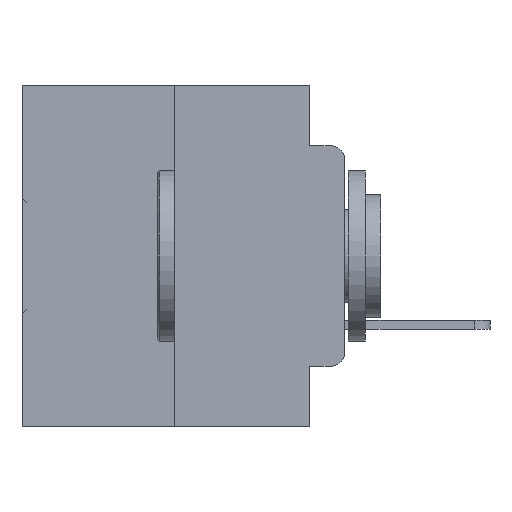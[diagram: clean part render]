
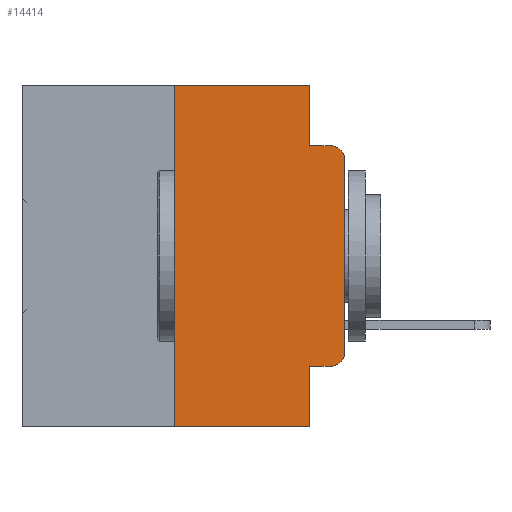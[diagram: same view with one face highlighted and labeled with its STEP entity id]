
A CAD part, left-side view. The second image highlights one B-rep face of the part: STEP entity #14414.
In plain terms, the highlighted planar face has unit normal (-1, 0, 0).
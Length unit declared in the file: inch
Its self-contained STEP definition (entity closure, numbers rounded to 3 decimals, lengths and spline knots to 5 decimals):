
#119 = EDGE_CURVE ( 'NONE', #28819, #12069, #9223, .T. ) ;
#246 = EDGE_CURVE ( 'NONE', #27324, #5881, #31484, .T. ) ;
#652 = VERTEX_POINT ( 'NONE', #22433 ) ;
#704 = EDGE_CURVE ( 'NONE', #30117, #28819, #18302, .T. ) ;
#799 = EDGE_CURVE ( 'NONE', #23162, #15607, #5548, .T. ) ;
#862 = EDGE_CURVE ( 'NONE', #652, #12604, #23609, .T. ) ;
#1151 = EDGE_CURVE ( 'NONE', #12604, #12069, #4268, .T. ) ;
#1583 = ORIENTED_EDGE ( 'NONE', *, *, #12006, .T. ) ;
#2366 = VECTOR ( 'NONE', #4319, 39.37008 ) ;
#2504 = VECTOR ( 'NONE', #8081, 39.37008 ) ;
#3049 = EDGE_CURVE ( 'NONE', #27824, #30117, #21275, .T. ) ;
#3473 = AXIS2_PLACEMENT_3D ( 'NONE', #25827, #9820, #28366 ) ;
#4268 = LINE ( 'NONE', #8154, #12706 ) ;
#4319 = DIRECTION ( 'NONE',  ( 0., -1., 0. ) ) ;
#5548 = LINE ( 'NONE', #22470, #20366 ) ;
#5781 = DIRECTION ( 'NONE',  ( -1., 0., 0. ) ) ;
#5881 = VERTEX_POINT ( 'NONE', #5897 ) ;
#5897 = CARTESIAN_POINT ( 'NONE',  ( 0., 0.051, -0.5 ) ) ;
#6065 = ORIENTED_EDGE ( 'NONE', *, *, #862, .F. ) ;
#6193 = AXIS2_PLACEMENT_3D ( 'NONE', #22319, #5781, #24837 ) ;
#8081 = DIRECTION ( 'NONE',  ( 0., 0., 1. ) ) ;
#8154 = CARTESIAN_POINT ( 'NONE',  ( 0., 0.051, -0.0885 ) ) ;
#8314 = ORIENTED_EDGE ( 'NONE', *, *, #119, .T. ) ;
#9223 = CIRCLE ( 'NONE', #25194, 0.02 ) ;
#9820 = DIRECTION ( 'NONE',  ( 1., 0., 0. ) ) ;
#9928 = LINE ( 'NONE', #9944, #2366 ) ;
#9944 = CARTESIAN_POINT ( 'NONE',  ( 0., 0.051, -0.4115 ) ) ;
#10684 = DIRECTION ( 'NONE',  ( 0., -1., 0. ) ) ;
#11235 = CARTESIAN_POINT ( 'NONE',  ( 0., 0.25, -0.5 ) ) ;
#11400 = CARTESIAN_POINT ( 'NONE',  ( 0., 0.051, 0. ) ) ;
#11892 = VECTOR ( 'NONE', #21802, 39.37008 ) ;
#12002 = FACE_OUTER_BOUND ( 'NONE', #21865, .T. ) ;
#12006 = EDGE_CURVE ( 'NONE', #23162, #5881, #20325, .T. ) ;
#12069 = VERTEX_POINT ( 'NONE', #24504 ) ;
#12518 = PLANE ( 'NONE',  #3473 ) ;
#12604 = VERTEX_POINT ( 'NONE', #28276 ) ;
#12706 = VECTOR ( 'NONE', #21235, 39.37008 ) ;
#13207 = EDGE_CURVE ( 'NONE', #15607, #652, #31679, .T. ) ;
#14011 = CARTESIAN_POINT ( 'NONE',  ( 0., 0., -0.3915 ) ) ;
#14414 = ADVANCED_FACE ( 'NONE', ( #12002 ), #12518, .F. ) ;
#15607 = VERTEX_POINT ( 'NONE', #29595 ) ;
#16439 = ORIENTED_EDGE ( 'NONE', *, *, #18289, .T. ) ;
#17074 = VECTOR ( 'NONE', #29434, 39.37008 ) ;
#17269 = VECTOR ( 'NONE', #23717, 39.37008 ) ;
#17514 = ORIENTED_EDGE ( 'NONE', *, *, #13207, .F. ) ;
#18289 = EDGE_CURVE ( 'NONE', #27324, #27824, #9928, .T. ) ;
#18302 = LINE ( 'NONE', #23955, #2504 ) ;
#19006 = CARTESIAN_POINT ( 'NONE',  ( 0., 0.473, -0.5 ) ) ;
#19931 = CARTESIAN_POINT ( 'NONE',  ( 0., 0., -0.1085 ) ) ;
#20325 = LINE ( 'NONE', #19006, #21122 ) ;
#20366 = VECTOR ( 'NONE', #30527, 39.37008 ) ;
#20840 = ORIENTED_EDGE ( 'NONE', *, *, #799, .F. ) ;
#21122 = VECTOR ( 'NONE', #10684, 39.37008 ) ;
#21148 = CARTESIAN_POINT ( 'NONE',  ( 0., 0.473, 0. ) ) ;
#21235 = DIRECTION ( 'NONE',  ( 0., -1., 0. ) ) ;
#21275 = CIRCLE ( 'NONE', #6193, 0.02 ) ;
#21577 = ORIENTED_EDGE ( 'NONE', *, *, #246, .F. ) ;
#21802 = DIRECTION ( 'NONE',  ( 0., 0., -1. ) ) ;
#21844 = DIRECTION ( 'NONE',  ( 0., 0., -1. ) ) ;
#21865 = EDGE_LOOP ( 'NONE', ( #28731, #8314, #29587, #6065, #17514, #20840, #1583, #21577, #16439, #25663 ) ) ;
#22099 = CARTESIAN_POINT ( 'NONE',  ( 0., 0.051, 0. ) ) ;
#22319 = CARTESIAN_POINT ( 'NONE',  ( 0., 0.02, -0.3915 ) ) ;
#22433 = CARTESIAN_POINT ( 'NONE',  ( 0., 0.051, 0. ) ) ;
#22470 = CARTESIAN_POINT ( 'NONE',  ( 0., 0.25, 0. ) ) ;
#23162 = VERTEX_POINT ( 'NONE', #11235 ) ;
#23609 = LINE ( 'NONE', #22099, #11892 ) ;
#23717 = DIRECTION ( 'NONE',  ( 0., -1., 0. ) ) ;
#23955 = CARTESIAN_POINT ( 'NONE',  ( 0., 0., 0. ) ) ;
#24005 = DIRECTION ( 'NONE',  ( -1., 0., 0. ) ) ;
#24504 = CARTESIAN_POINT ( 'NONE',  ( 0., 0.02, -0.0885 ) ) ;
#24837 = DIRECTION ( 'NONE',  ( 0., 0., -1. ) ) ;
#25194 = AXIS2_PLACEMENT_3D ( 'NONE', #26520, #24005, #21844 ) ;
#25663 = ORIENTED_EDGE ( 'NONE', *, *, #3049, .T. ) ;
#25827 = CARTESIAN_POINT ( 'NONE',  ( 0., 0.473, 0. ) ) ;
#26520 = CARTESIAN_POINT ( 'NONE',  ( 0., 0.02, -0.1085 ) ) ;
#27324 = VERTEX_POINT ( 'NONE', #29319 ) ;
#27824 = VERTEX_POINT ( 'NONE', #28520 ) ;
#28276 = CARTESIAN_POINT ( 'NONE',  ( 0., 0.051, -0.0885 ) ) ;
#28366 = DIRECTION ( 'NONE',  ( 0., 0., -1. ) ) ;
#28520 = CARTESIAN_POINT ( 'NONE',  ( 0., 0.02, -0.4115 ) ) ;
#28731 = ORIENTED_EDGE ( 'NONE', *, *, #704, .T. ) ;
#28819 = VERTEX_POINT ( 'NONE', #19931 ) ;
#29319 = CARTESIAN_POINT ( 'NONE',  ( 0., 0.051, -0.4115 ) ) ;
#29434 = DIRECTION ( 'NONE',  ( 0., 0., -1. ) ) ;
#29587 = ORIENTED_EDGE ( 'NONE', *, *, #1151, .F. ) ;
#29595 = CARTESIAN_POINT ( 'NONE',  ( 0., 0.25, 0. ) ) ;
#30117 = VERTEX_POINT ( 'NONE', #14011 ) ;
#30527 = DIRECTION ( 'NONE',  ( 0., 0., 1. ) ) ;
#31484 = LINE ( 'NONE', #11400, #17074 ) ;
#31679 = LINE ( 'NONE', #21148, #17269 ) ;
